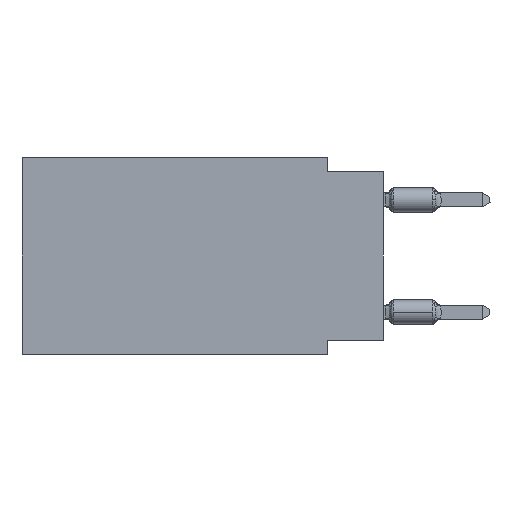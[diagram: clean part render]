
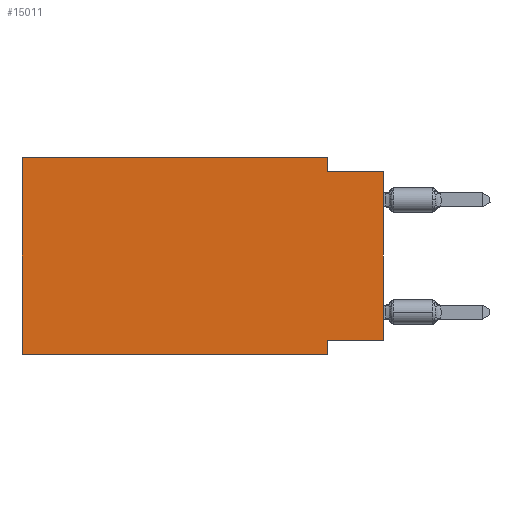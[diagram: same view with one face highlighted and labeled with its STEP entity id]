
A CAD part, left-side view. The second image highlights one B-rep face of the part: STEP entity #15011.
In plain terms, the highlighted planar face has unit normal (-1, 0, 0).
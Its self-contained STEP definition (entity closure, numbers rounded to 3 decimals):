
#75 = CARTESIAN_POINT ( 'NONE',  ( 0., 2.54, 0. ) ) ;
#318 = VERTEX_POINT ( 'NONE', #14010 ) ;
#423 = CARTESIAN_POINT ( 'NONE',  ( 0., 16.383, 0. ) ) ;
#932 = VERTEX_POINT ( 'NONE', #16677 ) ;
#1061 = ORIENTED_EDGE ( 'NONE', *, *, #22079, .T. ) ;
#2156 = EDGE_CURVE ( 'NONE', #15022, #17565, #18616, .T. ) ;
#2767 = CARTESIAN_POINT ( 'NONE',  ( 0., 0., -8.255 ) ) ;
#2772 = ORIENTED_EDGE ( 'NONE', *, *, #18345, .T. ) ;
#2805 = CARTESIAN_POINT ( 'NONE',  ( 0., 16.383, -8.89 ) ) ;
#3025 = VECTOR ( 'NONE', #19092, 1000. ) ;
#3130 = VECTOR ( 'NONE', #14742, 1000. ) ;
#3512 = DIRECTION ( 'NONE',  ( 0., 0., -1. ) ) ;
#3935 = CARTESIAN_POINT ( 'NONE',  ( 0., 16.383, -8.89 ) ) ;
#4155 = CARTESIAN_POINT ( 'NONE',  ( 0., 16.383, 0. ) ) ;
#4429 = EDGE_CURVE ( 'NONE', #12323, #318, #22917, .T. ) ;
#4471 = EDGE_CURVE ( 'NONE', #15934, #14973, #19962, .T. ) ;
#4813 = VECTOR ( 'NONE', #16476, 1000. ) ;
#5283 = CARTESIAN_POINT ( 'NONE',  ( 0., 0., -0.635 ) ) ;
#5369 = EDGE_LOOP ( 'NONE', ( #1061, #8091, #11917, #9850, #8870, #2772, #7880, #21121 ) ) ;
#5773 = DIRECTION ( 'NONE',  ( 1., 0., 0. ) ) ;
#5922 = LINE ( 'NONE', #11156, #13353 ) ;
#6418 = EDGE_CURVE ( 'NONE', #17565, #6779, #5922, .T. ) ;
#6694 = CARTESIAN_POINT ( 'NONE',  ( 0., 0., -8.255 ) ) ;
#6779 = VERTEX_POINT ( 'NONE', #5283 ) ;
#7544 = CARTESIAN_POINT ( 'NONE',  ( 0., 16.383, 0. ) ) ;
#7880 = ORIENTED_EDGE ( 'NONE', *, *, #21799, .F. ) ;
#7943 = DIRECTION ( 'NONE',  ( 0., -1., 0. ) ) ;
#8060 = CARTESIAN_POINT ( 'NONE',  ( 0., 2.54, 0. ) ) ;
#8091 = ORIENTED_EDGE ( 'NONE', *, *, #6418, .F. ) ;
#8188 = LINE ( 'NONE', #20864, #15749 ) ;
#8372 = LINE ( 'NONE', #2805, #8447 ) ;
#8447 = VECTOR ( 'NONE', #13471, 1000. ) ;
#8870 = ORIENTED_EDGE ( 'NONE', *, *, #4471, .F. ) ;
#9850 = ORIENTED_EDGE ( 'NONE', *, *, #11449, .F. ) ;
#11156 = CARTESIAN_POINT ( 'NONE',  ( 0., 0., -0.635 ) ) ;
#11189 = VECTOR ( 'NONE', #7943, 1000. ) ;
#11449 = EDGE_CURVE ( 'NONE', #14973, #15022, #22514, .T. ) ;
#11917 = ORIENTED_EDGE ( 'NONE', *, *, #2156, .F. ) ;
#12323 = VERTEX_POINT ( 'NONE', #2767 ) ;
#13044 = DIRECTION ( 'NONE',  ( 0., -1., 0. ) ) ;
#13110 = FACE_OUTER_BOUND ( 'NONE', #5369, .T. ) ;
#13353 = VECTOR ( 'NONE', #13044, 1000. ) ;
#13471 = DIRECTION ( 'NONE',  ( 0., -1., 0. ) ) ;
#14010 = CARTESIAN_POINT ( 'NONE',  ( 0., 2.54, -8.255 ) ) ;
#14742 = DIRECTION ( 'NONE',  ( 0., 0., 1. ) ) ;
#14973 = VERTEX_POINT ( 'NONE', #7544 ) ;
#15011 = ADVANCED_FACE ( 'NONE', ( #13110 ), #21884, .F. ) ;
#15022 = VERTEX_POINT ( 'NONE', #75 ) ;
#15749 = VECTOR ( 'NONE', #19109, 1000. ) ;
#15934 = VERTEX_POINT ( 'NONE', #3935 ) ;
#16007 = VECTOR ( 'NONE', #21143, 1000. ) ;
#16476 = DIRECTION ( 'NONE',  ( 0., 0., 1. ) ) ;
#16677 = CARTESIAN_POINT ( 'NONE',  ( 0., 2.54, -8.89 ) ) ;
#17550 = CARTESIAN_POINT ( 'NONE',  ( 0., 2.54, -0.635 ) ) ;
#17565 = VERTEX_POINT ( 'NONE', #17550 ) ;
#18091 = AXIS2_PLACEMENT_3D ( 'NONE', #423, #5773, #3512 ) ;
#18345 = EDGE_CURVE ( 'NONE', #15934, #932, #8372, .T. ) ;
#18616 = LINE ( 'NONE', #8060, #3025 ) ;
#19092 = DIRECTION ( 'NONE',  ( 0., 0., -1. ) ) ;
#19109 = DIRECTION ( 'NONE',  ( 0., 0., -1. ) ) ;
#19851 = CARTESIAN_POINT ( 'NONE',  ( 0., 16.383, 0. ) ) ;
#19962 = LINE ( 'NONE', #19851, #3130 ) ;
#20027 = CARTESIAN_POINT ( 'NONE',  ( 0., 0., 0. ) ) ;
#20864 = CARTESIAN_POINT ( 'NONE',  ( 0., 2.54, -8.89 ) ) ;
#21121 = ORIENTED_EDGE ( 'NONE', *, *, #4429, .F. ) ;
#21143 = DIRECTION ( 'NONE',  ( 0., 1., 0. ) ) ;
#21799 = EDGE_CURVE ( 'NONE', #318, #932, #8188, .T. ) ;
#21884 = PLANE ( 'NONE',  #18091 ) ;
#22079 = EDGE_CURVE ( 'NONE', #12323, #6779, #22144, .T. ) ;
#22144 = LINE ( 'NONE', #20027, #4813 ) ;
#22514 = LINE ( 'NONE', #4155, #11189 ) ;
#22917 = LINE ( 'NONE', #6694, #16007 ) ;
